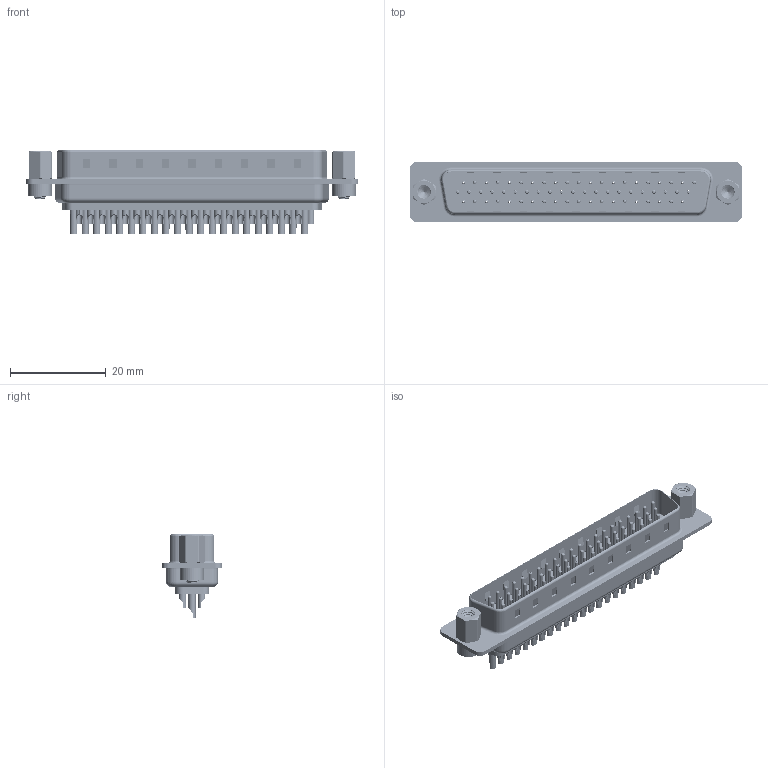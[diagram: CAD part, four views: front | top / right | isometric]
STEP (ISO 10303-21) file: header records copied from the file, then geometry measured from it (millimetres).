
FILE_DESCRIPTION (( 'STEP AP203' ), '1' );
FILE_NAME ('637-062-232-243.STEP', '2020-07-18T03:47:05', ( '' ), ( '' ), 'SwSTEP 2.0', 'SolidWorks 2020', '' );
FILE_SCHEMA (( 'CONFIG_CONTROL_DESIGN' ));
Length unit declared in the file: millimetre
Products named in the file (9): 637 Contact Row 3_32; 637 Contact Row 1_32; 637 Housing_62 Contacts; 637 Shell Rear_62 Contacts; 637 4-40 Hex Standoff; 637 4-40 Threaded Rivet; 637 Shell Front_62 Contacts; 637-062-232-243; 637 Contact Row 2_32
Assembly tree (69 placements, depth 2):
  637-062-232-243
    637 Housing_62 Contacts
    637 Shell Front_62 Contacts
    637 Shell Rear_62 Contacts
    637 Contact Row 1_32  x21
    637 Contact Row 2_32  x21
    637 Contact Row 3_32  x20
    637 4-40 Threaded Rivet  x2
    637 4-40 Hex Standoff  x2
Bounding box: 69.4 x 12.6 x 17.55 mm (x, y, z)
Volume: 3963 mm3; surface area: 14655.5 mm2
Topology: 69 solids, 69 shells, 4506 faces, 11573 edges, 7340 vertices
Faces by surface type: cylinder 2011, torus 1352, plane 1093, cone 32, bspline 18
Entity records: 40229 total; most frequent: CARTESIAN_POINT 10177, DIRECTION 6189, ORIENTED_EDGE 5404, EDGE_CURVE 2702, AXIS2_PLACEMENT_3D 2492, VERTEX_POINT 1747, EDGE_LOOP 1415, CIRCLE 1323
